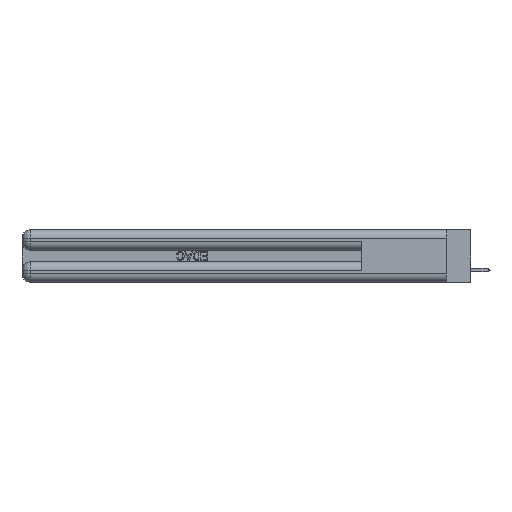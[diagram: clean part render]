
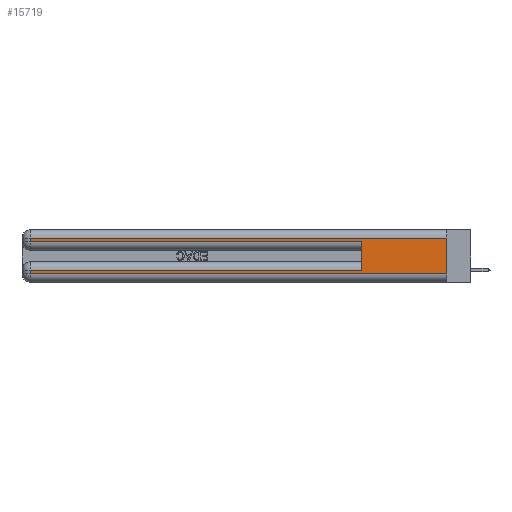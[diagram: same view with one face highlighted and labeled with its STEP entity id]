
A CAD part, left-side view. The second image highlights one B-rep face of the part: STEP entity #15719.
In plain terms, the highlighted planar face has unit normal (-1, 0, 0).
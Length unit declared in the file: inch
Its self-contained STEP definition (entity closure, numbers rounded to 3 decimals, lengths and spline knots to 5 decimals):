
#1254 = DIRECTION ( 'NONE',  ( 0., 0., -1. ) ) ;
#1560 = DIRECTION ( 'NONE',  ( 0., -1., 0. ) ) ;
#1739 = DIRECTION ( 'NONE',  ( 0., 0., -1. ) ) ;
#2244 = CARTESIAN_POINT ( 'NONE',  ( 0., 0.6, 0.285 ) ) ;
#2502 = VECTOR ( 'NONE', #1254, 39.37008 ) ;
#2952 = CARTESIAN_POINT ( 'NONE',  ( 0., 2.94, 0.37 ) ) ;
#3305 = CARTESIAN_POINT ( 'NONE',  ( 0., 2.94, 0.06 ) ) ;
#3323 = EDGE_CURVE ( 'NONE', #20787, #31144, #28241, .T. ) ;
#3477 = VECTOR ( 'NONE', #7609, 39.37008 ) ;
#3630 = LINE ( 'NONE', #20599, #37121 ) ;
#4902 = VERTEX_POINT ( 'NONE', #22538 ) ;
#5936 = EDGE_CURVE ( 'NONE', #32833, #39957, #3630, .T. ) ;
#6102 = ORIENTED_EDGE ( 'NONE', *, *, #6954, .T. ) ;
#6954 = EDGE_CURVE ( 'NONE', #4902, #29259, #40839, .T. ) ;
#7018 = CARTESIAN_POINT ( 'NONE',  ( 0., 0.6, 0.145 ) ) ;
#7609 = DIRECTION ( 'NONE',  ( 0., 0., 1. ) ) ;
#10253 = EDGE_CURVE ( 'NONE', #30219, #20787, #11362, .T. ) ;
#10454 = LINE ( 'NONE', #37516, #25747 ) ;
#10481 = CARTESIAN_POINT ( 'NONE',  ( 0., 0.6, 0.085 ) ) ;
#11005 = CARTESIAN_POINT ( 'NONE',  ( 0., 2.94, 0.37 ) ) ;
#11043 = PLANE ( 'NONE',  #21975 ) ;
#11362 = LINE ( 'NONE', #39927, #41763 ) ;
#13386 = VECTOR ( 'NONE', #39039, 39.37008 ) ;
#13863 = CARTESIAN_POINT ( 'NONE',  ( 0., 0., 0.37 ) ) ;
#14285 = FACE_OUTER_BOUND ( 'NONE', #41463, .T. ) ;
#14341 = DIRECTION ( 'NONE',  ( 0., 1., 0. ) ) ;
#15719 = ADVANCED_FACE ( 'NONE', ( #14285 ), #11043, .F. ) ;
#17078 = ORIENTED_EDGE ( 'NONE', *, *, #22724, .T. ) ;
#17628 = EDGE_CURVE ( 'NONE', #30219, #39957, #30925, .T. ) ;
#20599 = CARTESIAN_POINT ( 'NONE',  ( 0., 0., 0.285 ) ) ;
#20787 = VERTEX_POINT ( 'NONE', #30969 ) ;
#20799 = LINE ( 'NONE', #11005, #2502 ) ;
#21955 = CARTESIAN_POINT ( 'NONE',  ( 0., 2.94, 0.31 ) ) ;
#21975 = AXIS2_PLACEMENT_3D ( 'NONE', #40501, #24587, #1739 ) ;
#22538 = CARTESIAN_POINT ( 'NONE',  ( 0., 0., 0.31 ) ) ;
#22724 = EDGE_CURVE ( 'NONE', #29259, #32833, #20799, .T. ) ;
#24097 = DIRECTION ( 'NONE',  ( 0., 0., -1. ) ) ;
#24235 = DIRECTION ( 'NONE',  ( 0., -1., 0. ) ) ;
#24587 = DIRECTION ( 'NONE',  ( 1., 0., 0. ) ) ;
#25322 = ORIENTED_EDGE ( 'NONE', *, *, #25886, .T. ) ;
#25705 = CARTESIAN_POINT ( 'NONE',  ( 0., 0., 0.31 ) ) ;
#25747 = VECTOR ( 'NONE', #24235, 39.37008 ) ;
#25886 = EDGE_CURVE ( 'NONE', #31144, #38306, #10454, .T. ) ;
#27604 = ORIENTED_EDGE ( 'NONE', *, *, #38527, .F. ) ;
#28241 = LINE ( 'NONE', #2952, #40878 ) ;
#29259 = VERTEX_POINT ( 'NONE', #21955 ) ;
#30219 = VERTEX_POINT ( 'NONE', #10481 ) ;
#30925 = LINE ( 'NONE', #7018, #3477 ) ;
#30969 = CARTESIAN_POINT ( 'NONE',  ( 0., 2.94, 0.085 ) ) ;
#31144 = VERTEX_POINT ( 'NONE', #3305 ) ;
#32833 = VERTEX_POINT ( 'NONE', #40877 ) ;
#35728 = ORIENTED_EDGE ( 'NONE', *, *, #10253, .T. ) ;
#36714 = ORIENTED_EDGE ( 'NONE', *, *, #3323, .T. ) ;
#36905 = ORIENTED_EDGE ( 'NONE', *, *, #5936, .T. ) ;
#37121 = VECTOR ( 'NONE', #1560, 39.37008 ) ;
#37516 = CARTESIAN_POINT ( 'NONE',  ( 0., 0., 0.06 ) ) ;
#37937 = ORIENTED_EDGE ( 'NONE', *, *, #17628, .F. ) ;
#38306 = VERTEX_POINT ( 'NONE', #41543 ) ;
#38527 = EDGE_CURVE ( 'NONE', #4902, #38306, #39030, .T. ) ;
#38582 = VECTOR ( 'NONE', #24097, 39.37008 ) ;
#38630 = DIRECTION ( 'NONE',  ( 0., 0., -1. ) ) ;
#39030 = LINE ( 'NONE', #13863, #38582 ) ;
#39039 = DIRECTION ( 'NONE',  ( 0., 1., 0. ) ) ;
#39927 = CARTESIAN_POINT ( 'NONE',  ( 0., 0., 0.085 ) ) ;
#39957 = VERTEX_POINT ( 'NONE', #2244 ) ;
#40501 = CARTESIAN_POINT ( 'NONE',  ( 0., 0., 0.37 ) ) ;
#40839 = LINE ( 'NONE', #25705, #13386 ) ;
#40877 = CARTESIAN_POINT ( 'NONE',  ( 0., 2.94, 0.285 ) ) ;
#40878 = VECTOR ( 'NONE', #38630, 39.37008 ) ;
#41463 = EDGE_LOOP ( 'NONE', ( #27604, #6102, #17078, #36905, #37937, #35728, #36714, #25322 ) ) ;
#41543 = CARTESIAN_POINT ( 'NONE',  ( 0., 0., 0.06 ) ) ;
#41763 = VECTOR ( 'NONE', #14341, 39.37008 ) ;
